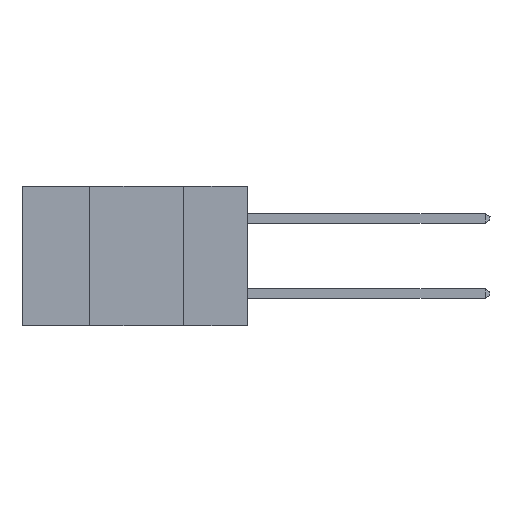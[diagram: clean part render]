
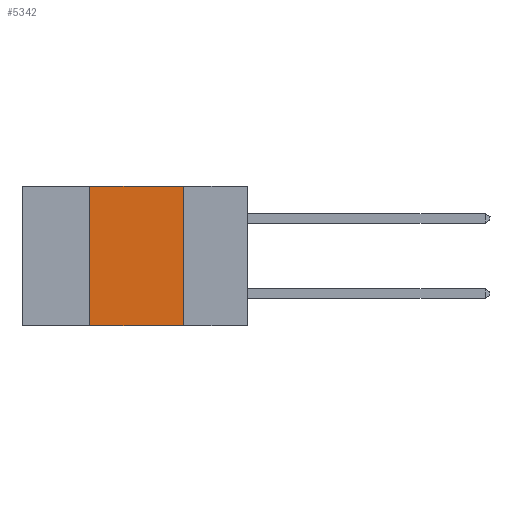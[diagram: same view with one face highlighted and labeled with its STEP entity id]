
A CAD part, left-side view. The second image highlights one B-rep face of the part: STEP entity #5342.
In plain terms, the highlighted planar face has unit normal (-1, 0, 0).
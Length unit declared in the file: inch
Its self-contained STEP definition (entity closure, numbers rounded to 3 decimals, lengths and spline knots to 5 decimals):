
#25 = CARTESIAN_POINT ( 'NONE',  ( 0., 0.17, 0. ) ) ;
#803 = VECTOR ( 'NONE', #19164, 39.37008 ) ;
#1568 = CARTESIAN_POINT ( 'NONE',  ( 0., 0.17, -0.37 ) ) ;
#1663 = DIRECTION ( 'NONE',  ( 0., 0., -1. ) ) ;
#2717 = LINE ( 'NONE', #7383, #11645 ) ;
#2952 = DIRECTION ( 'NONE',  ( 0., 0., 1. ) ) ;
#3250 = ORIENTED_EDGE ( 'NONE', *, *, #6055, .F. ) ;
#3657 = LINE ( 'NONE', #9939, #7470 ) ;
#3750 = ORIENTED_EDGE ( 'NONE', *, *, #19867, .T. ) ;
#4295 = EDGE_CURVE ( 'NONE', #18938, #16935, #2717, .T. ) ;
#4842 = VERTEX_POINT ( 'NONE', #18129 ) ;
#4928 = VERTEX_POINT ( 'NONE', #1568 ) ;
#5342 = ADVANCED_FACE ( 'NONE', ( #16534 ), #10662, .F. ) ;
#6055 = EDGE_CURVE ( 'NONE', #4842, #18938, #3657, .T. ) ;
#7383 = CARTESIAN_POINT ( 'NONE',  ( 0., 0.6, 0. ) ) ;
#7470 = VECTOR ( 'NONE', #2952, 39.37008 ) ;
#9177 = CARTESIAN_POINT ( 'NONE',  ( 0., 0.17, 0. ) ) ;
#9179 = DIRECTION ( 'NONE',  ( 0., -1., 0. ) ) ;
#9939 = CARTESIAN_POINT ( 'NONE',  ( 0., 0.42, 0. ) ) ;
#10662 = PLANE ( 'NONE',  #14325 ) ;
#11304 = EDGE_CURVE ( 'NONE', #16935, #4928, #17372, .T. ) ;
#11319 = CARTESIAN_POINT ( 'NONE',  ( 0., 0.6, -0.37 ) ) ;
#11645 = VECTOR ( 'NONE', #9179, 39.37008 ) ;
#13183 = VECTOR ( 'NONE', #1663, 39.37008 ) ;
#14043 = LINE ( 'NONE', #11319, #803 ) ;
#14205 = CARTESIAN_POINT ( 'NONE',  ( 0., 0.42, 0. ) ) ;
#14296 = DIRECTION ( 'NONE',  ( 1., 0., 0. ) ) ;
#14325 = AXIS2_PLACEMENT_3D ( 'NONE', #16491, #14296, #15451 ) ;
#14886 = ORIENTED_EDGE ( 'NONE', *, *, #11304, .F. ) ;
#15451 = DIRECTION ( 'NONE',  ( 0., 0., -1. ) ) ;
#16491 = CARTESIAN_POINT ( 'NONE',  ( 0., 0.6, 0. ) ) ;
#16534 = FACE_OUTER_BOUND ( 'NONE', #17300, .T. ) ;
#16935 = VERTEX_POINT ( 'NONE', #9177 ) ;
#17300 = EDGE_LOOP ( 'NONE', ( #14886, #19479, #3250, #3750 ) ) ;
#17372 = LINE ( 'NONE', #25, #13183 ) ;
#18129 = CARTESIAN_POINT ( 'NONE',  ( 0., 0.42, -0.37 ) ) ;
#18938 = VERTEX_POINT ( 'NONE', #14205 ) ;
#19164 = DIRECTION ( 'NONE',  ( 0., -1., 0. ) ) ;
#19479 = ORIENTED_EDGE ( 'NONE', *, *, #4295, .F. ) ;
#19867 = EDGE_CURVE ( 'NONE', #4842, #4928, #14043, .T. ) ;
